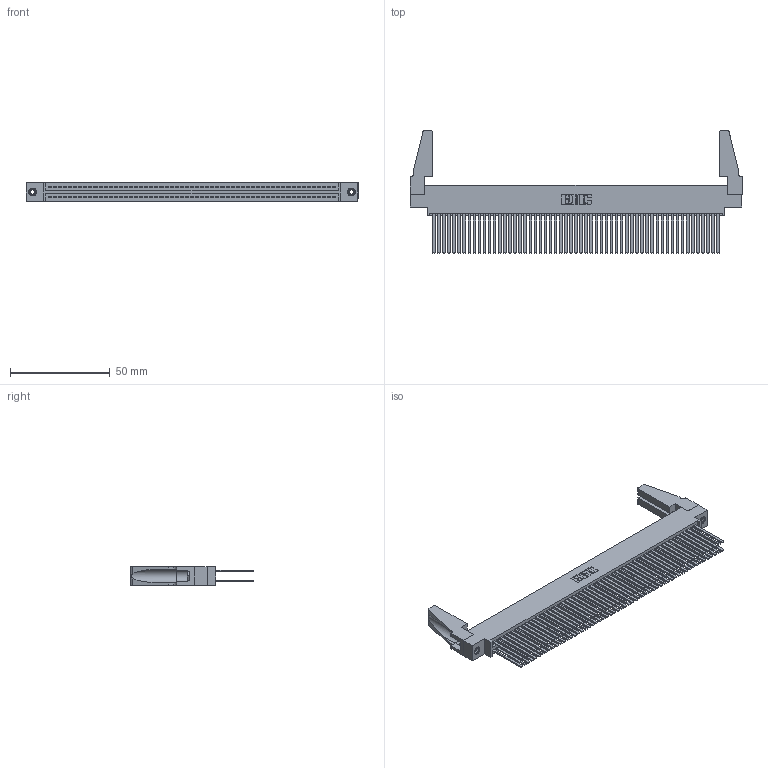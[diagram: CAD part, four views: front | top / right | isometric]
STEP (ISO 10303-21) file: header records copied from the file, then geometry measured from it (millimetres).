
FILE_DESCRIPTION (( 'STEP AP203' ), '1' );
FILE_NAME ('395-114-544-888.STEP', '2019-10-27T18:41:58', ( '' ), ( '' ), 'SwSTEP 2.0', 'SolidWorks 2016', '' );
FILE_SCHEMA (( 'CONFIG_CONTROL_DESIGN' ));
Length unit declared in the file: inch
Products named in the file (5): 345-250-001_345-250-001-102; 345-220-078_345-220-088; 395-114-544-888; 345 Part_0.170 Offset - 0.156 Dia-TH; 345-292-001_345-293-144
Assembly tree (119 placements, depth 2):
  395-114-544-888
    345 Part_0.170 Offset - 0.156 Dia-TH
    345-292-001_345-293-144  x114
    345-250-001_345-250-001-102  x2
    345-220-078_345-220-088  x2
Bounding box: 166.01 x 61.14 x 9.4 mm (x, y, z)
Volume: 21003.2 mm3; surface area: 34478.5 mm2
Topology: 119 solids, 119 shells, 5270 faces, 15601 edges, 10238 vertices
Faces by surface type: plane 3462, cylinder 1792, cone 12, torus 4
Entity records: 44800 total; most frequent: CARTESIAN_POINT 7490, ORIENTED_EDGE 7384, DIRECTION 6588, EDGE_CURVE 3692, VECTOR 3294, LINE 3294, VERTEX_POINT 2454, AXIS2_PLACEMENT_3D 1647
